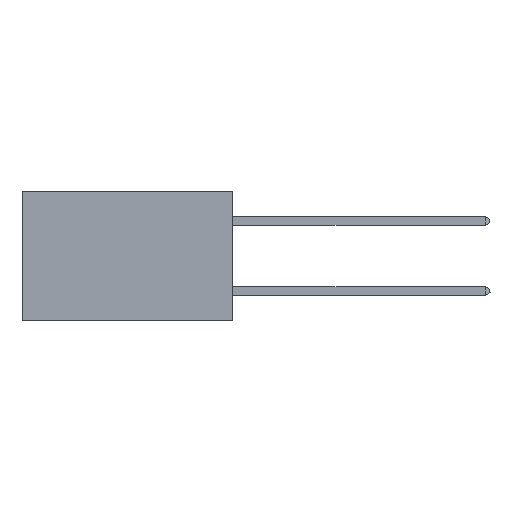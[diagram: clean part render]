
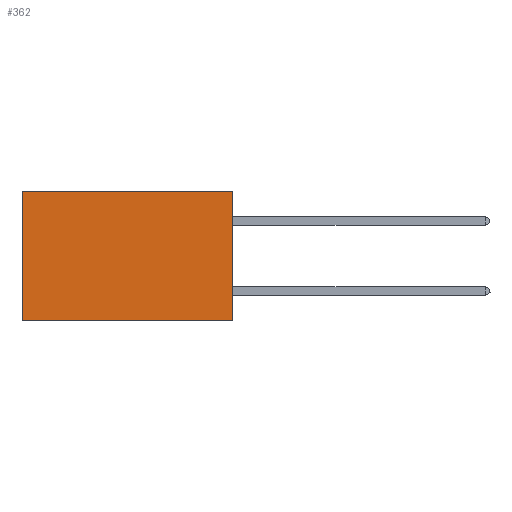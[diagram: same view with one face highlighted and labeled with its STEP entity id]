
A CAD part, left-side view. The second image highlights one B-rep face of the part: STEP entity #362.
In plain terms, the highlighted planar face has unit normal (-1, 0, 0).
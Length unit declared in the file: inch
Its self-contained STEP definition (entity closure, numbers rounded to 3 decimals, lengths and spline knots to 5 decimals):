
#336 = LINE ( 'NONE', #2359, #7766 ) ;
#362 = ADVANCED_FACE ( 'NONE', ( #1630 ), #1506, .F. ) ;
#413 = VERTEX_POINT ( 'NONE', #8767 ) ;
#735 = DIRECTION ( 'NONE',  ( 0., 0., -1. ) ) ;
#766 = DIRECTION ( 'NONE',  ( 0., 0., -1. ) ) ;
#939 = LINE ( 'NONE', #3260, #7627 ) ;
#1473 = LINE ( 'NONE', #2490, #8545 ) ;
#1506 = PLANE ( 'NONE',  #6516 ) ;
#1538 = CARTESIAN_POINT ( 'NONE',  ( 0.2875, 0., 0. ) ) ;
#1630 = FACE_OUTER_BOUND ( 'NONE', #6399, .T. ) ;
#1994 = CARTESIAN_POINT ( 'NONE',  ( 0.2875, 0.6, 0. ) ) ;
#2147 = VERTEX_POINT ( 'NONE', #1994 ) ;
#2273 = CARTESIAN_POINT ( 'NONE',  ( 0.2875, 0., 0. ) ) ;
#2348 = ORIENTED_EDGE ( 'NONE', *, *, #6321, .T. ) ;
#2359 = CARTESIAN_POINT ( 'NONE',  ( 0.2875, 0., -0.37 ) ) ;
#2490 = CARTESIAN_POINT ( 'NONE',  ( 0.2875, 0.6, 0. ) ) ;
#3106 = CARTESIAN_POINT ( 'NONE',  ( 0.2875, 0.6, -0.37 ) ) ;
#3260 = CARTESIAN_POINT ( 'NONE',  ( 0.2875, 0., 0. ) ) ;
#3858 = DIRECTION ( 'NONE',  ( 1., 0., 0. ) ) ;
#4113 = LINE ( 'NONE', #1538, #7906 ) ;
#4605 = DIRECTION ( 'NONE',  ( 0., 0., -1. ) ) ;
#4836 = VERTEX_POINT ( 'NONE', #3106 ) ;
#4921 = EDGE_CURVE ( 'NONE', #2147, #4836, #1473, .T. ) ;
#6242 = EDGE_CURVE ( 'NONE', #413, #4836, #336, .T. ) ;
#6321 = EDGE_CURVE ( 'NONE', #7334, #2147, #939, .T. ) ;
#6399 = EDGE_LOOP ( 'NONE', ( #8094, #9184, #7551, #2348 ) ) ;
#6516 = AXIS2_PLACEMENT_3D ( 'NONE', #2273, #3858, #4605 ) ;
#7090 = DIRECTION ( 'NONE',  ( 0., 1., 0. ) ) ;
#7334 = VERTEX_POINT ( 'NONE', #8885 ) ;
#7415 = DIRECTION ( 'NONE',  ( 0., 1., 0. ) ) ;
#7551 = ORIENTED_EDGE ( 'NONE', *, *, #7909, .F. ) ;
#7627 = VECTOR ( 'NONE', #7415, 39.37008 ) ;
#7766 = VECTOR ( 'NONE', #7090, 39.37008 ) ;
#7906 = VECTOR ( 'NONE', #735, 39.37008 ) ;
#7909 = EDGE_CURVE ( 'NONE', #7334, #413, #4113, .T. ) ;
#8094 = ORIENTED_EDGE ( 'NONE', *, *, #4921, .T. ) ;
#8545 = VECTOR ( 'NONE', #766, 39.37008 ) ;
#8767 = CARTESIAN_POINT ( 'NONE',  ( 0.2875, 0., -0.37 ) ) ;
#8885 = CARTESIAN_POINT ( 'NONE',  ( 0.2875, 0., 0. ) ) ;
#9184 = ORIENTED_EDGE ( 'NONE', *, *, #6242, .F. ) ;
